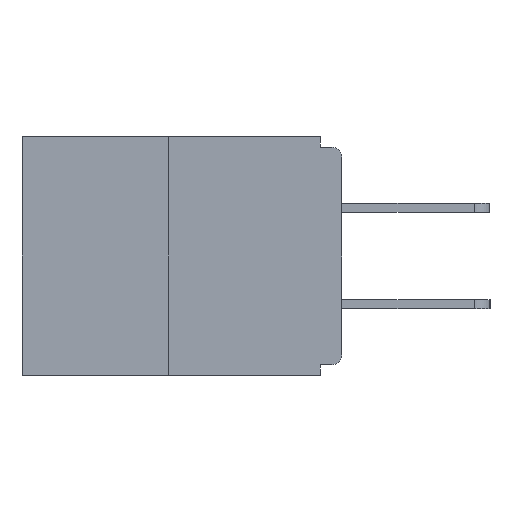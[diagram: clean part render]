
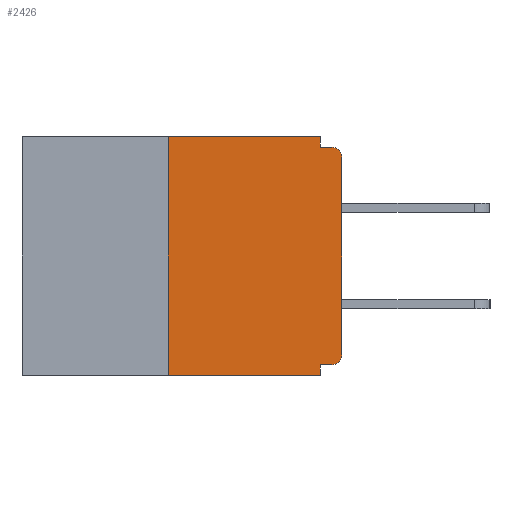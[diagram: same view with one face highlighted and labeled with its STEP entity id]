
A CAD part, left-side view. The second image highlights one B-rep face of the part: STEP entity #2426.
In plain terms, the highlighted planar face has unit normal (-1, 0, 0).
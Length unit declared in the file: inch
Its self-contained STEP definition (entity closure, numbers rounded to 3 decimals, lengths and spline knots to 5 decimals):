
#791 = DIRECTION ( 'NONE',  ( 0., 0., -1. ) ) ;
#962 = VERTEX_POINT ( 'NONE', #9542 ) ;
#1055 = EDGE_CURVE ( 'NONE', #962, #7386, #7762, .T. ) ;
#1141 = VERTEX_POINT ( 'NONE', #10558 ) ;
#1167 = EDGE_CURVE ( 'NONE', #4799, #3476, #12874, .T. ) ;
#1849 = EDGE_CURVE ( 'NONE', #5616, #2806, #3029, .T. ) ;
#1956 = EDGE_LOOP ( 'NONE', ( #3618, #8493, #7010, #10984, #7591, #4886, #12369, #6550, #11243, #8406 ) ) ;
#2057 = VECTOR ( 'NONE', #791, 39.37008 ) ;
#2125 = LINE ( 'NONE', #4198, #9890 ) ;
#2406 = CARTESIAN_POINT ( 'NONE',  ( 0., 0., -0.328 ) ) ;
#2426 = ADVANCED_FACE ( 'NONE', ( #5053 ), #2931, .F. ) ;
#2477 = CARTESIAN_POINT ( 'NONE',  ( 0., 0.46, 0. ) ) ;
#2726 = VECTOR ( 'NONE', #6522, 39.37008 ) ;
#2806 = VERTEX_POINT ( 'NONE', #11739 ) ;
#2931 = PLANE ( 'NONE',  #10453 ) ;
#3029 = CIRCLE ( 'NONE', #8752, 0.015 ) ;
#3208 = DIRECTION ( 'NONE',  ( 0., -1., 0. ) ) ;
#3323 = VECTOR ( 'NONE', #3968, 39.37008 ) ;
#3476 = VERTEX_POINT ( 'NONE', #9770 ) ;
#3475 = LINE ( 'NONE', #2477, #2726 ) ;
#3521 = VECTOR ( 'NONE', #10641, 39.37008 ) ;
#3618 = ORIENTED_EDGE ( 'NONE', *, *, #10173, .F. ) ;
#3771 = EDGE_CURVE ( 'NONE', #11276, #7386, #10775, .T. ) ;
#3800 = DIRECTION ( 'NONE',  ( 0., 0., 1. ) ) ;
#3968 = DIRECTION ( 'NONE',  ( 0., 0., -1. ) ) ;
#4124 = DIRECTION ( 'NONE',  ( 0., 0., 1. ) ) ;
#4198 = CARTESIAN_POINT ( 'NONE',  ( 0., 0., 0. ) ) ;
#4250 = CARTESIAN_POINT ( 'NONE',  ( 0., 0.015, -0.03 ) ) ;
#4278 = VECTOR ( 'NONE', #3800, 39.37008 ) ;
#4474 = LINE ( 'NONE', #2406, #3521 ) ;
#4555 = CARTESIAN_POINT ( 'NONE',  ( 0., 0.015, -0.313 ) ) ;
#4799 = VERTEX_POINT ( 'NONE', #7519 ) ;
#4886 = ORIENTED_EDGE ( 'NONE', *, *, #1849, .T. ) ;
#5052 = AXIS2_PLACEMENT_3D ( 'NONE', #4250, #6227, #6302 ) ;
#5053 = FACE_OUTER_BOUND ( 'NONE', #1956, .T. ) ;
#5110 = VECTOR ( 'NONE', #10620, 39.37008 ) ;
#5278 = VERTEX_POINT ( 'NONE', #6417 ) ;
#5607 = DIRECTION ( 'NONE',  ( -1., 0., 0. ) ) ;
#5616 = VERTEX_POINT ( 'NONE', #12180 ) ;
#5812 = CARTESIAN_POINT ( 'NONE',  ( 0., 0.031, -0.343 ) ) ;
#6100 = DIRECTION ( 'NONE',  ( 1., 0., 0. ) ) ;
#6104 = EDGE_CURVE ( 'NONE', #4799, #5278, #9974, .T. ) ;
#6227 = DIRECTION ( 'NONE',  ( -1., 0., 0. ) ) ;
#6302 = DIRECTION ( 'NONE',  ( 0., 0., -1. ) ) ;
#6372 = EDGE_CURVE ( 'NONE', #5616, #1141, #4474, .T. ) ;
#6417 = CARTESIAN_POINT ( 'NONE',  ( 0., 0.031, -0.343 ) ) ;
#6522 = DIRECTION ( 'NONE',  ( 0., -1., 0. ) ) ;
#6550 = ORIENTED_EDGE ( 'NONE', *, *, #3771, .T. ) ;
#6567 = CARTESIAN_POINT ( 'NONE',  ( 0., 0., -0.015 ) ) ;
#6823 = CARTESIAN_POINT ( 'NONE',  ( 0., 0., -0.03 ) ) ;
#7010 = ORIENTED_EDGE ( 'NONE', *, *, #6104, .T. ) ;
#7072 = CARTESIAN_POINT ( 'NONE',  ( 0., 0.031, 0. ) ) ;
#7284 = EDGE_CURVE ( 'NONE', #12716, #962, #12190, .T. ) ;
#7386 = VERTEX_POINT ( 'NONE', #10395 ) ;
#7519 = CARTESIAN_POINT ( 'NONE',  ( 0., 0.25, -0.343 ) ) ;
#7523 = DIRECTION ( 'NONE',  ( 0., 0., -1. ) ) ;
#7591 = ORIENTED_EDGE ( 'NONE', *, *, #6372, .F. ) ;
#7714 = EDGE_CURVE ( 'NONE', #1141, #5278, #10931, .T. ) ;
#7762 = LINE ( 'NONE', #6567, #5110 ) ;
#7828 = CARTESIAN_POINT ( 'NONE',  ( 0., 0.25, 0. ) ) ;
#8086 = CARTESIAN_POINT ( 'NONE',  ( 0., 0.46, 0. ) ) ;
#8406 = ORIENTED_EDGE ( 'NONE', *, *, #7284, .F. ) ;
#8493 = ORIENTED_EDGE ( 'NONE', *, *, #1167, .F. ) ;
#8752 = AXIS2_PLACEMENT_3D ( 'NONE', #4555, #5607, #7523 ) ;
#8893 = DIRECTION ( 'NONE',  ( 0., 0., -1. ) ) ;
#9374 = CARTESIAN_POINT ( 'NONE',  ( 0., 0.46, -0.343 ) ) ;
#9542 = CARTESIAN_POINT ( 'NONE',  ( 0., 0.031, -0.015 ) ) ;
#9770 = CARTESIAN_POINT ( 'NONE',  ( 0., 0.25, 0. ) ) ;
#9890 = VECTOR ( 'NONE', #4124, 39.37008 ) ;
#9974 = LINE ( 'NONE', #9374, #11558 ) ;
#10173 = EDGE_CURVE ( 'NONE', #3476, #12716, #3475, .T. ) ;
#10395 = CARTESIAN_POINT ( 'NONE',  ( 0., 0.015, -0.015 ) ) ;
#10453 = AXIS2_PLACEMENT_3D ( 'NONE', #8086, #6100, #8893 ) ;
#10558 = CARTESIAN_POINT ( 'NONE',  ( 0., 0.031, -0.328 ) ) ;
#10620 = DIRECTION ( 'NONE',  ( 0., -1., 0. ) ) ;
#10641 = DIRECTION ( 'NONE',  ( 0., 1., 0. ) ) ;
#10775 = CIRCLE ( 'NONE', #5052, 0.015 ) ;
#10931 = LINE ( 'NONE', #5812, #3323 ) ;
#10984 = ORIENTED_EDGE ( 'NONE', *, *, #7714, .F. ) ;
#11226 = CARTESIAN_POINT ( 'NONE',  ( 0., 0.031, 0. ) ) ;
#11243 = ORIENTED_EDGE ( 'NONE', *, *, #1055, .F. ) ;
#11276 = VERTEX_POINT ( 'NONE', #6823 ) ;
#11558 = VECTOR ( 'NONE', #3208, 39.37008 ) ;
#11739 = CARTESIAN_POINT ( 'NONE',  ( 0., 0., -0.313 ) ) ;
#12180 = CARTESIAN_POINT ( 'NONE',  ( 0., 0.015, -0.328 ) ) ;
#12190 = LINE ( 'NONE', #7072, #2057 ) ;
#12369 = ORIENTED_EDGE ( 'NONE', *, *, #12952, .T. ) ;
#12716 = VERTEX_POINT ( 'NONE', #11226 ) ;
#12874 = LINE ( 'NONE', #7828, #4278 ) ;
#12952 = EDGE_CURVE ( 'NONE', #2806, #11276, #2125, .T. ) ;
